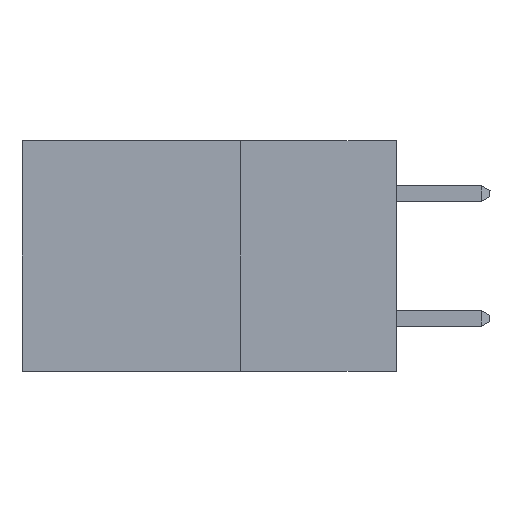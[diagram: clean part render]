
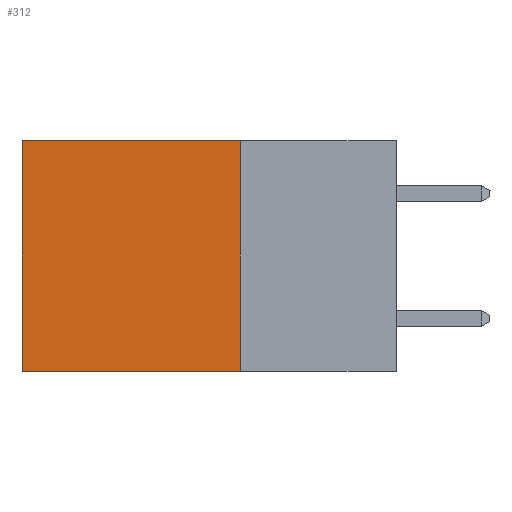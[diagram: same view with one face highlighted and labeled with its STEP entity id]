
A CAD part, left-side view. The second image highlights one B-rep face of the part: STEP entity #312.
In plain terms, the highlighted planar face has unit normal (-1, 0, 0).
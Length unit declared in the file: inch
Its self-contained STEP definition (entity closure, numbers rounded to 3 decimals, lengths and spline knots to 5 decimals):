
#312 = ADVANCED_FACE ( 'NONE', ( #6881 ), #4066, .F. ) ;
#366 = LINE ( 'NONE', #4702, #3907 ) ;
#564 = CARTESIAN_POINT ( 'NONE',  ( 0.298, 0.6, -0.37 ) ) ;
#1173 = DIRECTION ( 'NONE',  ( 0., 1., 0. ) ) ;
#1326 = VECTOR ( 'NONE', #4263, 39.37008 ) ;
#2023 = ORIENTED_EDGE ( 'NONE', *, *, #5752, .F. ) ;
#2656 = LINE ( 'NONE', #4072, #4420 ) ;
#2953 = ORIENTED_EDGE ( 'NONE', *, *, #4929, .T. ) ;
#3109 = VERTEX_POINT ( 'NONE', #6523 ) ;
#3357 = VECTOR ( 'NONE', #3867, 39.37008 ) ;
#3657 = LINE ( 'NONE', #7011, #1326 ) ;
#3852 = VERTEX_POINT ( 'NONE', #8316 ) ;
#3867 = DIRECTION ( 'NONE',  ( 0., 1., 0. ) ) ;
#3907 = VECTOR ( 'NONE', #1173, 39.37008 ) ;
#4066 = PLANE ( 'NONE',  #8504 ) ;
#4072 = CARTESIAN_POINT ( 'NONE',  ( 0.298, 0.25, 0. ) ) ;
#4263 = DIRECTION ( 'NONE',  ( 0., 0., -1. ) ) ;
#4294 = EDGE_CURVE ( 'NONE', #3109, #4657, #3657, .T. ) ;
#4420 = VECTOR ( 'NONE', #10228, 39.37008 ) ;
#4460 = VERTEX_POINT ( 'NONE', #7425 ) ;
#4657 = VERTEX_POINT ( 'NONE', #564 ) ;
#4702 = CARTESIAN_POINT ( 'NONE',  ( 0.298, 0.25, 0. ) ) ;
#4851 = DIRECTION ( 'NONE',  ( 1., 0., 0. ) ) ;
#4929 = EDGE_CURVE ( 'NONE', #3852, #3109, #366, .T. ) ;
#5752 = EDGE_CURVE ( 'NONE', #3852, #4460, #2656, .T. ) ;
#6416 = CARTESIAN_POINT ( 'NONE',  ( 0.298, 0.25, -0.37 ) ) ;
#6523 = CARTESIAN_POINT ( 'NONE',  ( 0.298, 0.6, 0. ) ) ;
#6673 = CARTESIAN_POINT ( 'NONE',  ( 0.298, 0.25, 0. ) ) ;
#6769 = ORIENTED_EDGE ( 'NONE', *, *, #10512, .F. ) ;
#6881 = FACE_OUTER_BOUND ( 'NONE', #7802, .T. ) ;
#7011 = CARTESIAN_POINT ( 'NONE',  ( 0.298, 0.6, 0. ) ) ;
#7108 = ORIENTED_EDGE ( 'NONE', *, *, #4294, .T. ) ;
#7425 = CARTESIAN_POINT ( 'NONE',  ( 0.298, 0.25, -0.37 ) ) ;
#7802 = EDGE_LOOP ( 'NONE', ( #7108, #6769, #2023, #2953 ) ) ;
#8316 = CARTESIAN_POINT ( 'NONE',  ( 0.298, 0.25, 0. ) ) ;
#8366 = DIRECTION ( 'NONE',  ( 0., 0., -1. ) ) ;
#8504 = AXIS2_PLACEMENT_3D ( 'NONE', #6673, #4851, #8366 ) ;
#10228 = DIRECTION ( 'NONE',  ( 0., 0., -1. ) ) ;
#10512 = EDGE_CURVE ( 'NONE', #4460, #4657, #11091, .T. ) ;
#11091 = LINE ( 'NONE', #6416, #3357 ) ;
